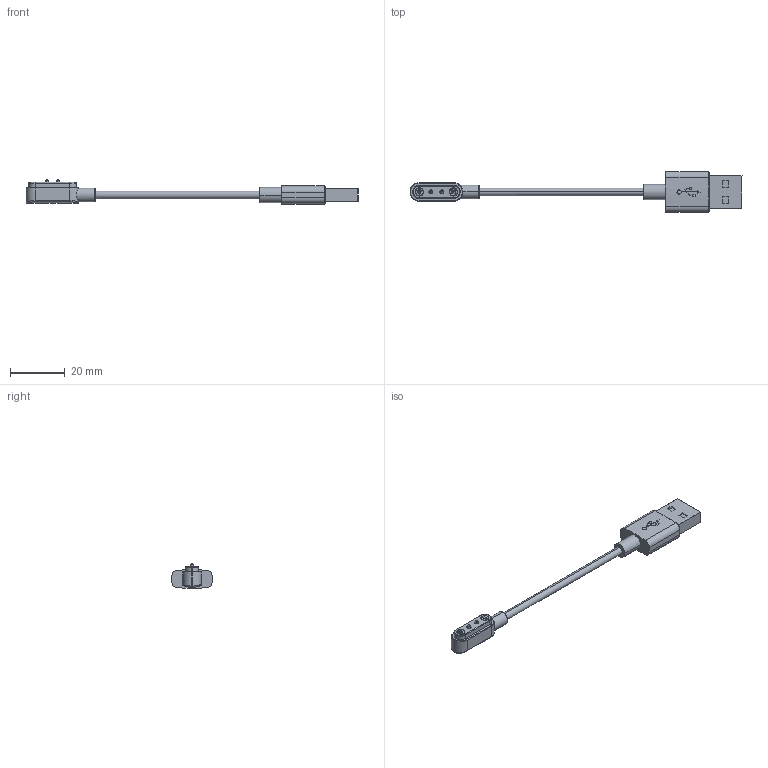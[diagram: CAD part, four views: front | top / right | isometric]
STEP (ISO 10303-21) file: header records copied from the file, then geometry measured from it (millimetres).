
FILE_DESCRIPTION (( 'STEP AP203' ), '1' );
FILE_NAME ('687-L0222A111200.STEP', '2023-02-11T06:57:11', ( '' ), ( '' ), 'SwSTEP 2.0', 'SolidWorks 2020', '' );
FILE_SCHEMA (( 'CONFIG_CONTROL_DESIGN' ));
Length unit declared in the file: millimetre
Products named in the file (1): 687-L0222A111200
Bounding box: 121.03 x 14.8 x 8.95 mm (x, y, z)
Surface area: 3448.1 mm2 (no closed solid volume)
Topology: 0 solids, 8 shells, 324 faces, 775 edges, 494 vertices
Faces by surface type: plane 149, cylinder 112, torus 25, bspline 21, cone 17
Entity records: 11563 total; most frequent: CARTESIAN_POINT 4313, ORIENTED_EDGE 1538, DIRECTION 1366, EDGE_CURVE 771, AXIS2_PLACEMENT_3D 519, VERTEX_POINT 494, EDGE_LOOP 371, LINE 328
